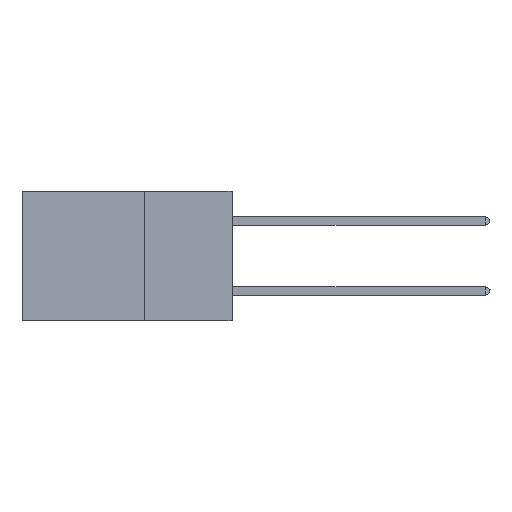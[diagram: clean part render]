
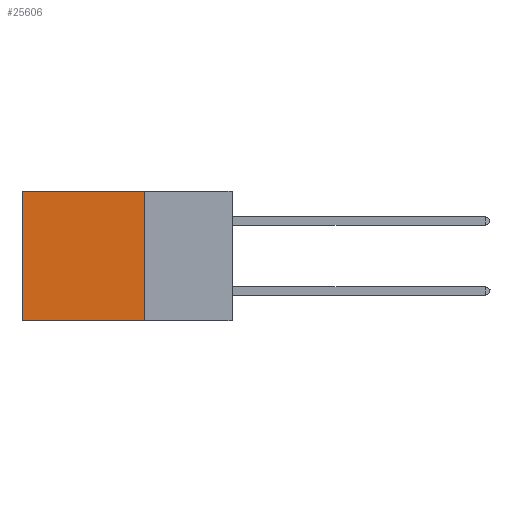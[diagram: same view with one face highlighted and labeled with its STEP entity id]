
A CAD part, left-side view. The second image highlights one B-rep face of the part: STEP entity #25606.
In plain terms, the highlighted planar face has unit normal (-1, 0, 0).
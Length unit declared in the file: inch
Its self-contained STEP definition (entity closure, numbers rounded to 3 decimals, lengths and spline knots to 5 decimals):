
#411 = AXIS2_PLACEMENT_3D ( 'NONE', #25393, #28544, #9529 ) ;
#1335 = VECTOR ( 'NONE', #25023, 39.37008 ) ;
#1622 = CARTESIAN_POINT ( 'NONE',  ( 0.2875, 0.6, 0. ) ) ;
#2508 = DIRECTION ( 'NONE',  ( 0., 0., -1. ) ) ;
#7189 = EDGE_CURVE ( 'NONE', #28975, #7740, #26486, .T. ) ;
#7740 = VERTEX_POINT ( 'NONE', #10960 ) ;
#8320 = LINE ( 'NONE', #37313, #16266 ) ;
#8507 = VECTOR ( 'NONE', #25101, 39.37008 ) ;
#9529 = DIRECTION ( 'NONE',  ( 0., 0., -1. ) ) ;
#9909 = EDGE_CURVE ( 'NONE', #28710, #7740, #8320, .T. ) ;
#10584 = DIRECTION ( 'NONE',  ( 0., 1., 0. ) ) ;
#10960 = CARTESIAN_POINT ( 'NONE',  ( 0.2875, 0.6, -0.37 ) ) ;
#12201 = ORIENTED_EDGE ( 'NONE', *, *, #9909, .T. ) ;
#13520 = VECTOR ( 'NONE', #10584, 39.37008 ) ;
#15146 = ORIENTED_EDGE ( 'NONE', *, *, #34726, .F. ) ;
#16266 = VECTOR ( 'NONE', #2508, 39.37008 ) ;
#20309 = ORIENTED_EDGE ( 'NONE', *, *, #7189, .F. ) ;
#20608 = VERTEX_POINT ( 'NONE', #35775 ) ;
#21945 = PLANE ( 'NONE',  #411 ) ;
#22114 = CARTESIAN_POINT ( 'NONE',  ( 0.2875, 0.25, 0. ) ) ;
#25023 = DIRECTION ( 'NONE',  ( 0., 1., 0. ) ) ;
#25101 = DIRECTION ( 'NONE',  ( 0., 0., -1. ) ) ;
#25393 = CARTESIAN_POINT ( 'NONE',  ( 0.2875, 0.25, 0. ) ) ;
#25606 = ADVANCED_FACE ( 'NONE', ( #40135 ), #21945, .F. ) ;
#26486 = LINE ( 'NONE', #32956, #13520 ) ;
#26544 = ORIENTED_EDGE ( 'NONE', *, *, #37047, .T. ) ;
#28544 = DIRECTION ( 'NONE',  ( 1., 0., 0. ) ) ;
#28710 = VERTEX_POINT ( 'NONE', #1622 ) ;
#28975 = VERTEX_POINT ( 'NONE', #29415 ) ;
#29415 = CARTESIAN_POINT ( 'NONE',  ( 0.2875, 0.25, -0.37 ) ) ;
#32956 = CARTESIAN_POINT ( 'NONE',  ( 0.2875, 0.25, -0.37 ) ) ;
#34726 = EDGE_CURVE ( 'NONE', #20608, #28975, #40347, .T. ) ;
#35699 = LINE ( 'NONE', #22114, #1335 ) ;
#35775 = CARTESIAN_POINT ( 'NONE',  ( 0.2875, 0.25, 0. ) ) ;
#36593 = EDGE_LOOP ( 'NONE', ( #12201, #20309, #15146, #26544 ) ) ;
#37047 = EDGE_CURVE ( 'NONE', #20608, #28710, #35699, .T. ) ;
#37313 = CARTESIAN_POINT ( 'NONE',  ( 0.2875, 0.6, 0. ) ) ;
#40135 = FACE_OUTER_BOUND ( 'NONE', #36593, .T. ) ;
#40347 = LINE ( 'NONE', #40409, #8507 ) ;
#40409 = CARTESIAN_POINT ( 'NONE',  ( 0.2875, 0.25, 0. ) ) ;
